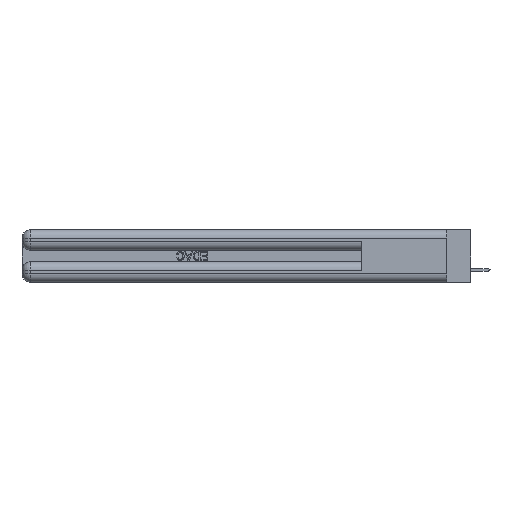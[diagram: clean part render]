
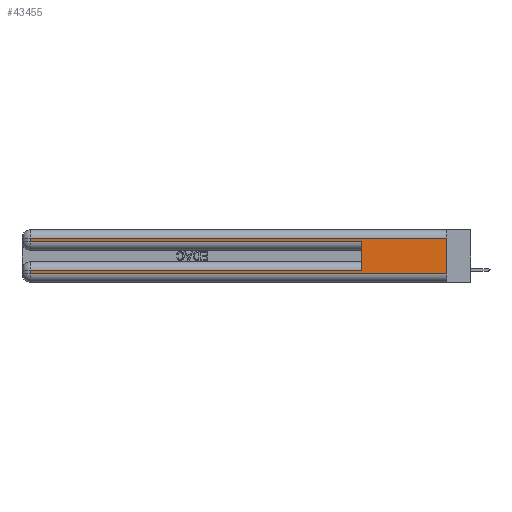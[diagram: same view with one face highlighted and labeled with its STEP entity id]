
A CAD part, left-side view. The second image highlights one B-rep face of the part: STEP entity #43455.
In plain terms, the highlighted planar face has unit normal (-1, 0, 0).
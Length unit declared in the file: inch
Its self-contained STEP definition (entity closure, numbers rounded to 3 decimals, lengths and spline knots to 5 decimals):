
#20 = CARTESIAN_POINT ( 'NONE',  ( 0., 0.6, 0.145 ) ) ;
#284 = CARTESIAN_POINT ( 'NONE',  ( 0., 0.6, 0.085 ) ) ;
#834 = EDGE_CURVE ( 'NONE', #37505, #22793, #4975, .T. ) ;
#1159 = DIRECTION ( 'NONE',  ( 0., 0., -1. ) ) ;
#2160 = VECTOR ( 'NONE', #34840, 39.37008 ) ;
#3232 = CARTESIAN_POINT ( 'NONE',  ( 0., 2.94, 0.06 ) ) ;
#3685 = CARTESIAN_POINT ( 'NONE',  ( 0., 0., 0.31 ) ) ;
#3703 = ORIENTED_EDGE ( 'NONE', *, *, #16407, .T. ) ;
#4476 = EDGE_LOOP ( 'NONE', ( #12189, #3703, #28364, #42176, #42385, #27705, #30077, #8336 ) ) ;
#4538 = CARTESIAN_POINT ( 'NONE',  ( 0., 2.94, 0.37 ) ) ;
#4975 = LINE ( 'NONE', #4538, #10320 ) ;
#4989 = VERTEX_POINT ( 'NONE', #284 ) ;
#6305 = CARTESIAN_POINT ( 'NONE',  ( 0., 2.94, 0.285 ) ) ;
#6882 = LINE ( 'NONE', #13213, #20121 ) ;
#7914 = LINE ( 'NONE', #3685, #26862 ) ;
#8336 = ORIENTED_EDGE ( 'NONE', *, *, #38955, .T. ) ;
#9229 = DIRECTION ( 'NONE',  ( 0., 1., 0. ) ) ;
#9255 = EDGE_CURVE ( 'NONE', #26108, #31446, #39727, .T. ) ;
#9378 = CARTESIAN_POINT ( 'NONE',  ( 0., 0., 0.37 ) ) ;
#9463 = VERTEX_POINT ( 'NONE', #19950 ) ;
#10320 = VECTOR ( 'NONE', #1159, 39.37008 ) ;
#10837 = VECTOR ( 'NONE', #29204, 39.37008 ) ;
#12189 = ORIENTED_EDGE ( 'NONE', *, *, #43386, .F. ) ;
#13213 = CARTESIAN_POINT ( 'NONE',  ( 0., 0., 0.37 ) ) ;
#13436 = PLANE ( 'NONE',  #15129 ) ;
#13776 = LINE ( 'NONE', #38680, #22173 ) ;
#14162 = CARTESIAN_POINT ( 'NONE',  ( 0., 0., 0.06 ) ) ;
#15129 = AXIS2_PLACEMENT_3D ( 'NONE', #9378, #30518, #43973 ) ;
#16407 = EDGE_CURVE ( 'NONE', #34095, #26108, #7914, .T. ) ;
#17411 = DIRECTION ( 'NONE',  ( 0., 1., 0. ) ) ;
#18924 = CARTESIAN_POINT ( 'NONE',  ( 0., 0.6, 0.285 ) ) ;
#19950 = CARTESIAN_POINT ( 'NONE',  ( 0., 0., 0.06 ) ) ;
#20072 = DIRECTION ( 'NONE',  ( 0., 0., 1. ) ) ;
#20121 = VECTOR ( 'NONE', #37030, 39.37008 ) ;
#20255 = CARTESIAN_POINT ( 'NONE',  ( 0., 0., 0.085 ) ) ;
#22173 = VECTOR ( 'NONE', #41162, 39.37008 ) ;
#22793 = VERTEX_POINT ( 'NONE', #3232 ) ;
#23824 = EDGE_CURVE ( 'NONE', #31446, #27534, #13776, .T. ) ;
#24269 = EDGE_CURVE ( 'NONE', #4989, #37505, #40022, .T. ) ;
#25682 = CARTESIAN_POINT ( 'NONE',  ( 0., 2.94, 0.085 ) ) ;
#26108 = VERTEX_POINT ( 'NONE', #35461 ) ;
#26862 = VECTOR ( 'NONE', #17411, 39.37008 ) ;
#27221 = LINE ( 'NONE', #14162, #2160 ) ;
#27534 = VERTEX_POINT ( 'NONE', #18924 ) ;
#27705 = ORIENTED_EDGE ( 'NONE', *, *, #24269, .T. ) ;
#28364 = ORIENTED_EDGE ( 'NONE', *, *, #9255, .T. ) ;
#29204 = DIRECTION ( 'NONE',  ( 0., 0., -1. ) ) ;
#30077 = ORIENTED_EDGE ( 'NONE', *, *, #834, .T. ) ;
#30518 = DIRECTION ( 'NONE',  ( 1., 0., 0. ) ) ;
#31163 = EDGE_CURVE ( 'NONE', #4989, #27534, #37357, .T. ) ;
#31446 = VERTEX_POINT ( 'NONE', #6305 ) ;
#32129 = CARTESIAN_POINT ( 'NONE',  ( 0., 2.94, 0.37 ) ) ;
#34095 = VERTEX_POINT ( 'NONE', #36744 ) ;
#34840 = DIRECTION ( 'NONE',  ( 0., -1., 0. ) ) ;
#35461 = CARTESIAN_POINT ( 'NONE',  ( 0., 2.94, 0.31 ) ) ;
#36744 = CARTESIAN_POINT ( 'NONE',  ( 0., 0., 0.31 ) ) ;
#37030 = DIRECTION ( 'NONE',  ( 0., 0., -1. ) ) ;
#37357 = LINE ( 'NONE', #20, #40545 ) ;
#37505 = VERTEX_POINT ( 'NONE', #25682 ) ;
#38680 = CARTESIAN_POINT ( 'NONE',  ( 0., 0., 0.285 ) ) ;
#38955 = EDGE_CURVE ( 'NONE', #22793, #9463, #27221, .T. ) ;
#39727 = LINE ( 'NONE', #32129, #10837 ) ;
#40022 = LINE ( 'NONE', #20255, #41537 ) ;
#40545 = VECTOR ( 'NONE', #20072, 39.37008 ) ;
#41162 = DIRECTION ( 'NONE',  ( 0., -1., 0. ) ) ;
#41537 = VECTOR ( 'NONE', #9229, 39.37008 ) ;
#42176 = ORIENTED_EDGE ( 'NONE', *, *, #23824, .T. ) ;
#42385 = ORIENTED_EDGE ( 'NONE', *, *, #31163, .F. ) ;
#43386 = EDGE_CURVE ( 'NONE', #34095, #9463, #6882, .T. ) ;
#43455 = ADVANCED_FACE ( 'NONE', ( #44407 ), #13436, .F. ) ;
#43973 = DIRECTION ( 'NONE',  ( 0., 0., -1. ) ) ;
#44407 = FACE_OUTER_BOUND ( 'NONE', #4476, .T. ) ;
